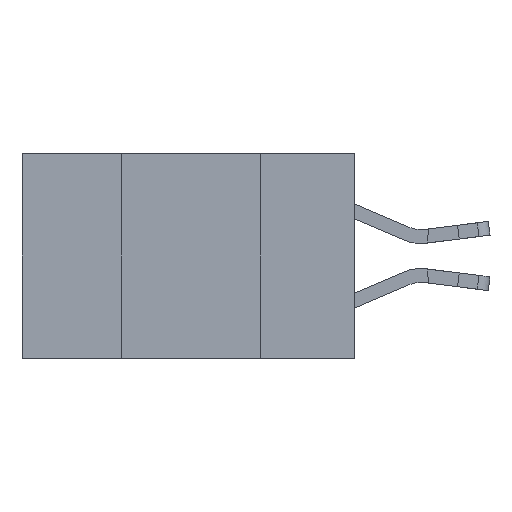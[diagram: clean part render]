
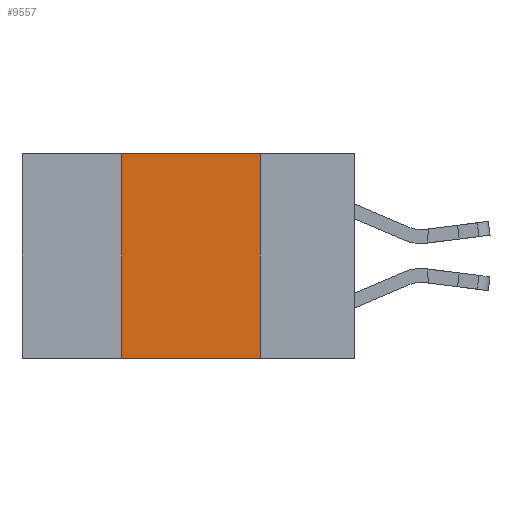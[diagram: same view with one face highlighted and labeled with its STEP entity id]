
A CAD part, left-side view. The second image highlights one B-rep face of the part: STEP entity #9557.
In plain terms, the highlighted planar face has unit normal (-1, 0, 0).
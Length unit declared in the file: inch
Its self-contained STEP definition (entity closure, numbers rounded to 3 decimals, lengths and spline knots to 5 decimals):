
#369 = CARTESIAN_POINT ( 'NONE',  ( 0., 0.6, 0. ) ) ;
#589 = VECTOR ( 'NONE', #9324, 39.37008 ) ;
#721 = VERTEX_POINT ( 'NONE', #11302 ) ;
#793 = EDGE_LOOP ( 'NONE', ( #2538, #2800, #2691, #4700 ) ) ;
#1133 = LINE ( 'NONE', #7970, #7192 ) ;
#1441 = VERTEX_POINT ( 'NONE', #9849 ) ;
#1579 = VERTEX_POINT ( 'NONE', #2064 ) ;
#2064 = CARTESIAN_POINT ( 'NONE',  ( 0., 0.17, -0.37 ) ) ;
#2538 = ORIENTED_EDGE ( 'NONE', *, *, #8299, .F. ) ;
#2691 = ORIENTED_EDGE ( 'NONE', *, *, #3849, .F. ) ;
#2800 = ORIENTED_EDGE ( 'NONE', *, *, #6527, .F. ) ;
#3849 = EDGE_CURVE ( 'NONE', #721, #1441, #11040, .T. ) ;
#4391 = LINE ( 'NONE', #369, #10438 ) ;
#4530 = DIRECTION ( 'NONE',  ( 0., -1., 0. ) ) ;
#4700 = ORIENTED_EDGE ( 'NONE', *, *, #6190, .T. ) ;
#5874 = CARTESIAN_POINT ( 'NONE',  ( 0., 0.42, 0. ) ) ;
#6031 = PLANE ( 'NONE',  #7995 ) ;
#6190 = EDGE_CURVE ( 'NONE', #721, #1579, #1133, .T. ) ;
#6527 = EDGE_CURVE ( 'NONE', #1441, #15594, #4391, .T. ) ;
#6606 = DIRECTION ( 'NONE',  ( 0., 0., -1. ) ) ;
#7192 = VECTOR ( 'NONE', #4530, 39.37008 ) ;
#7198 = DIRECTION ( 'NONE',  ( 0., 0., -1. ) ) ;
#7411 = CARTESIAN_POINT ( 'NONE',  ( 0., 0.17, 0. ) ) ;
#7970 = CARTESIAN_POINT ( 'NONE',  ( 0., 0.6, -0.37 ) ) ;
#7995 = AXIS2_PLACEMENT_3D ( 'NONE', #10844, #14416, #7198 ) ;
#8299 = EDGE_CURVE ( 'NONE', #15594, #1579, #13154, .T. ) ;
#9324 = DIRECTION ( 'NONE',  ( 0., 0., 1. ) ) ;
#9557 = ADVANCED_FACE ( 'NONE', ( #14820 ), #6031, .F. ) ;
#9849 = CARTESIAN_POINT ( 'NONE',  ( 0., 0.42, 0. ) ) ;
#9991 = VECTOR ( 'NONE', #6606, 39.37008 ) ;
#10438 = VECTOR ( 'NONE', #15304, 39.37008 ) ;
#10844 = CARTESIAN_POINT ( 'NONE',  ( 0., 0.6, 0. ) ) ;
#11040 = LINE ( 'NONE', #5874, #589 ) ;
#11302 = CARTESIAN_POINT ( 'NONE',  ( 0., 0.42, -0.37 ) ) ;
#13154 = LINE ( 'NONE', #13749, #9991 ) ;
#13749 = CARTESIAN_POINT ( 'NONE',  ( 0., 0.17, 0. ) ) ;
#14416 = DIRECTION ( 'NONE',  ( 1., 0., 0. ) ) ;
#14820 = FACE_OUTER_BOUND ( 'NONE', #793, .T. ) ;
#15304 = DIRECTION ( 'NONE',  ( 0., -1., 0. ) ) ;
#15594 = VERTEX_POINT ( 'NONE', #7411 ) ;
